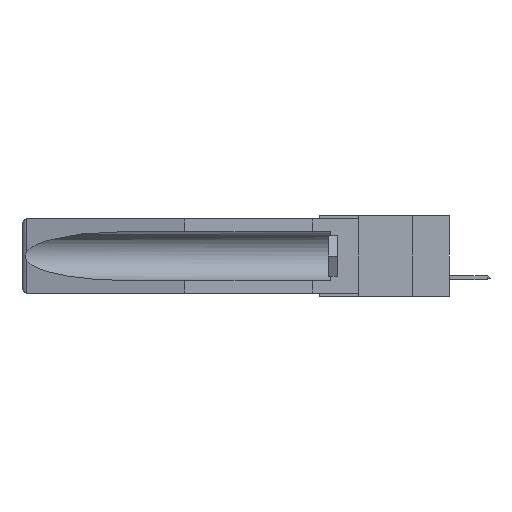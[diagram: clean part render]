
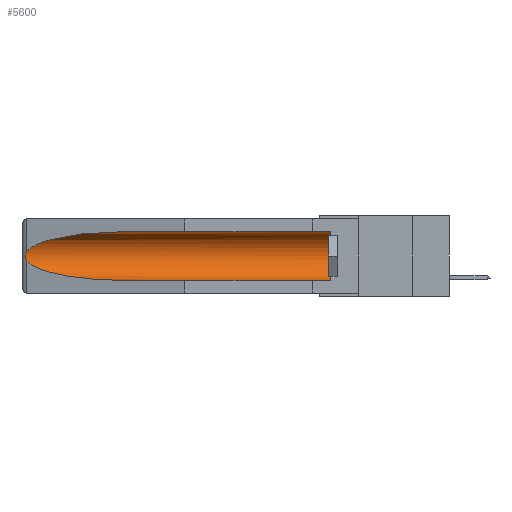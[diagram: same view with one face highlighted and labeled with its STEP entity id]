
A CAD part, left-side view. The second image highlights one B-rep face of the part: STEP entity #5600.
In plain terms, the highlighted cylindrical face has radius 2.857 mm (diameter 5.715 mm), a partial arc.
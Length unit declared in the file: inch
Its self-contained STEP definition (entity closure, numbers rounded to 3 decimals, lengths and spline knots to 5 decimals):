
#160 = VERTEX_POINT ( 'NONE', #16777 ) ;
#212 = VERTEX_POINT ( 'NONE', #1093 ) ;
#570 = EDGE_CURVE ( 'NONE', #212, #17206, #20087, .T. ) ;
#639 = CARTESIAN_POINT ( 'NONE',  ( 0.21114, 1.30732, -0.059 ) ) ;
#717 = DIRECTION ( 'NONE',  ( 0., 0., 1. ) ) ;
#1093 = CARTESIAN_POINT ( 'NONE',  ( 0.155, 0.126, -0.284 ) ) ;
#1150 = VERTEX_POINT ( 'NONE', #22476 ) ;
#1774 = CARTESIAN_POINT ( 'NONE',  ( 0.155, -0.30754, -0.284 ) ) ;
#2269 = FACE_OUTER_BOUND ( 'NONE', #5073, .T. ) ;
#2641 = CARTESIAN_POINT ( 'NONE',  ( 0.26537, 1.52718, -0.14972 ) ) ;
#3295 = AXIS2_PLACEMENT_3D ( 'NONE', #21967, #22037, #717 ) ;
#3583 = LINE ( 'NONE', #13084, #5251 ) ;
#4236 = DIRECTION ( 'NONE',  ( 0., 1., 0. ) ) ;
#4444 = VERTEX_POINT ( 'NONE', #19946 ) ;
#4526 =( BOUNDED_CURVE ( )  B_SPLINE_CURVE ( 3, ( #5826, #639, #19939, #2641 ),
 .UNSPECIFIED., .F., .F. ) 
 B_SPLINE_CURVE_WITH_KNOTS ( ( 4, 4 ),
 ( 4.71239, 6.08839 ),
 .UNSPECIFIED. ) 
 CURVE ( )  GEOMETRIC_REPRESENTATION_ITEM ( )  RATIONAL_B_SPLINE_CURVE ( ( 1., 0.848, 0.848, 1. ) ) 
 REPRESENTATION_ITEM ( '' )  );
#5009 = CYLINDRICAL_SURFACE ( 'NONE', #3295, 0.1125 ) ;
#5073 = EDGE_LOOP ( 'NONE', ( #20308, #22069, #20125, #14006, #9057, #12560 ) ) ;
#5251 = VECTOR ( 'NONE', #4236, 39.37008 ) ;
#5473 = VERTEX_POINT ( 'NONE', #21515 ) ;
#5503 = DIRECTION ( 'NONE',  ( 0., -1., 0. ) ) ;
#5600 = ADVANCED_FACE ( 'NONE', ( #2269 ), #5009, .F. ) ;
#5611 = B_SPLINE_CURVE_WITH_KNOTS ( 'NONE', 3,
 ( #17575, #12051, #22822, #13794, #17414, #20971, #13866, #10353, #21127, #22739 ),
 .UNSPECIFIED., .F., .F.,
 ( 4, 2, 2, 2, 4 ),
 ( 0., 0.00029, 0.00058, 0.00087, 0.00117 ),
 .UNSPECIFIED. ) ;
#5826 = CARTESIAN_POINT ( 'NONE',  ( 0.155, 1.07973, -0.059 ) ) ;
#7345 = DIRECTION ( 'NONE',  ( 0., 0., 1. ) ) ;
#7743 = EDGE_CURVE ( 'NONE', #212, #4444, #21135, .T. ) ;
#9057 = ORIENTED_EDGE ( 'NONE', *, *, #7743, .T. ) ;
#10353 = CARTESIAN_POINT ( 'NONE',  ( 0.26655, 1.53094, -0.18657 ) ) ;
#10826 = EDGE_CURVE ( 'NONE', #5473, #17206, #11527, .T. ) ;
#11527 =( BOUNDED_CURVE ( )  B_SPLINE_CURVE ( 3, ( #11585, #18871, #13549, #11821 ),
 .UNSPECIFIED., .F., .F. ) 
 B_SPLINE_CURVE_WITH_KNOTS ( ( 4, 4 ),
 ( 0.1948, 1.5708 ),
 .UNSPECIFIED. ) 
 CURVE ( )  GEOMETRIC_REPRESENTATION_ITEM ( )  RATIONAL_B_SPLINE_CURVE ( ( 1., 0.848, 0.848, 1. ) ) 
 REPRESENTATION_ITEM ( '' )  );
#11585 = CARTESIAN_POINT ( 'NONE',  ( 0.26537, 1.52718, -0.19328 ) ) ;
#11723 = AXIS2_PLACEMENT_3D ( 'NONE', #17925, #5503, #7345 ) ;
#11821 = CARTESIAN_POINT ( 'NONE',  ( 0.155, 1.07973, -0.284 ) ) ;
#12051 = CARTESIAN_POINT ( 'NONE',  ( 0.26597, 1.52961, -0.15275 ) ) ;
#12560 = ORIENTED_EDGE ( 'NONE', *, *, #19528, .T. ) ;
#13084 = CARTESIAN_POINT ( 'NONE',  ( 0.155, -0.30754, -0.059 ) ) ;
#13549 = CARTESIAN_POINT ( 'NONE',  ( 0.21114, 1.30732, -0.284 ) ) ;
#13794 = CARTESIAN_POINT ( 'NONE',  ( 0.2673, 1.5327, -0.16383 ) ) ;
#13866 = CARTESIAN_POINT ( 'NONE',  ( 0.2673, 1.53269, -0.17917 ) ) ;
#14006 = ORIENTED_EDGE ( 'NONE', *, *, #570, .F. ) ;
#15678 = EDGE_CURVE ( 'NONE', #1150, #5473, #5611, .T. ) ;
#16285 = DIRECTION ( 'NONE',  ( 0., 1., 0. ) ) ;
#16777 = CARTESIAN_POINT ( 'NONE',  ( 0.155, 1.07973, -0.059 ) ) ;
#17206 = VERTEX_POINT ( 'NONE', #21162 ) ;
#17414 = CARTESIAN_POINT ( 'NONE',  ( 0.2675, 1.53308, -0.16763 ) ) ;
#17575 = CARTESIAN_POINT ( 'NONE',  ( 0.26537, 1.52718, -0.14972 ) ) ;
#17925 = CARTESIAN_POINT ( 'NONE',  ( 0.155, 0.126, -0.1715 ) ) ;
#18153 = VECTOR ( 'NONE', #16285, 39.37008 ) ;
#18871 = CARTESIAN_POINT ( 'NONE',  ( 0.25451, 1.48313, -0.24835 ) ) ;
#19528 = EDGE_CURVE ( 'NONE', #4444, #160, #3583, .T. ) ;
#19939 = CARTESIAN_POINT ( 'NONE',  ( 0.25451, 1.48313, -0.09465 ) ) ;
#19946 = CARTESIAN_POINT ( 'NONE',  ( 0.155, 0.126, -0.059 ) ) ;
#20087 = LINE ( 'NONE', #1774, #18153 ) ;
#20125 = ORIENTED_EDGE ( 'NONE', *, *, #10826, .T. ) ;
#20308 = ORIENTED_EDGE ( 'NONE', *, *, #22272, .T. ) ;
#20971 = CARTESIAN_POINT ( 'NONE',  ( 0.2675, 1.53308, -0.17534 ) ) ;
#21127 = CARTESIAN_POINT ( 'NONE',  ( 0.26597, 1.5296, -0.19026 ) ) ;
#21135 = CIRCLE ( 'NONE', #11723, 0.1125 ) ;
#21162 = CARTESIAN_POINT ( 'NONE',  ( 0.155, 1.07973, -0.284 ) ) ;
#21515 = CARTESIAN_POINT ( 'NONE',  ( 0.26537, 1.52718, -0.19328 ) ) ;
#21967 = CARTESIAN_POINT ( 'NONE',  ( 0.155, -0.30754, -0.1715 ) ) ;
#22037 = DIRECTION ( 'NONE',  ( 0., 1., 0. ) ) ;
#22069 = ORIENTED_EDGE ( 'NONE', *, *, #15678, .T. ) ;
#22272 = EDGE_CURVE ( 'NONE', #160, #1150, #4526, .T. ) ;
#22476 = CARTESIAN_POINT ( 'NONE',  ( 0.26537, 1.52718, -0.14972 ) ) ;
#22739 = CARTESIAN_POINT ( 'NONE',  ( 0.26537, 1.52718, -0.19328 ) ) ;
#22822 = CARTESIAN_POINT ( 'NONE',  ( 0.26654, 1.53092, -0.15636 ) ) ;
